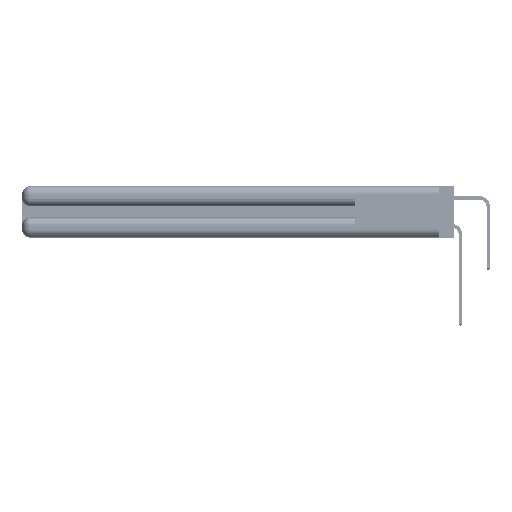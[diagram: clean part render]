
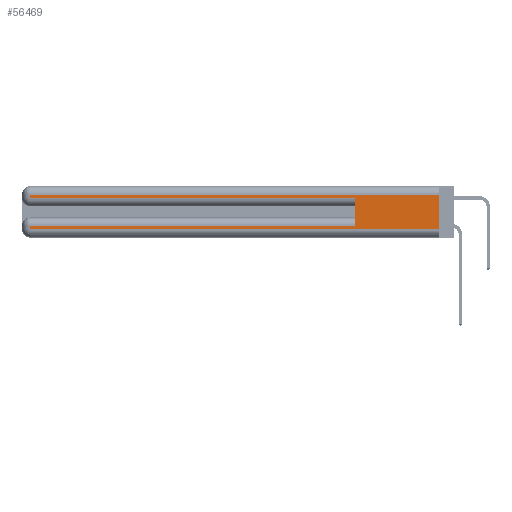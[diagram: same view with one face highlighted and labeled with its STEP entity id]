
A CAD part, left-side view. The second image highlights one B-rep face of the part: STEP entity #56469.
In plain terms, the highlighted planar face has unit normal (-1, 0, 0).
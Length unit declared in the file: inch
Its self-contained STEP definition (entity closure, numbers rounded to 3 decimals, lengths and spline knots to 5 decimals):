
#226 = VECTOR ( 'NONE', #22528, 39.37008 ) ;
#577 = CARTESIAN_POINT ( 'NONE',  ( 0., 0., 0.31 ) ) ;
#932 = CARTESIAN_POINT ( 'NONE',  ( 0., 0., 0.31 ) ) ;
#1440 = ORIENTED_EDGE ( 'NONE', *, *, #50047, .T. ) ;
#1702 = DIRECTION ( 'NONE',  ( 0., 0., -1. ) ) ;
#3631 = CARTESIAN_POINT ( 'NONE',  ( 0., 2.94, 0.37 ) ) ;
#4319 = DIRECTION ( 'NONE',  ( 0., -1., 0. ) ) ;
#5588 = ORIENTED_EDGE ( 'NONE', *, *, #55265, .F. ) ;
#5700 = DIRECTION ( 'NONE',  ( 0., 1., 0. ) ) ;
#7514 = CARTESIAN_POINT ( 'NONE',  ( 0., 0.6, 0.085 ) ) ;
#7896 = VERTEX_POINT ( 'NONE', #24627 ) ;
#8628 = DIRECTION ( 'NONE',  ( 0., 0., -1. ) ) ;
#9315 = CARTESIAN_POINT ( 'NONE',  ( 0., 2.94, 0.31 ) ) ;
#9508 = VERTEX_POINT ( 'NONE', #26844 ) ;
#10034 = EDGE_CURVE ( 'NONE', #7896, #24308, #26933, .T. ) ;
#10511 = LINE ( 'NONE', #32100, #226 ) ;
#11722 = CARTESIAN_POINT ( 'NONE',  ( 0., 0., 0.085 ) ) ;
#12884 = EDGE_CURVE ( 'NONE', #9508, #7896, #23349, .T. ) ;
#13428 = EDGE_LOOP ( 'NONE', ( #24247, #50853, #1440, #20833, #5588, #23877, #18763, #14285 ) ) ;
#14285 = ORIENTED_EDGE ( 'NONE', *, *, #10034, .T. ) ;
#14536 = FACE_OUTER_BOUND ( 'NONE', #13428, .T. ) ;
#16169 = VERTEX_POINT ( 'NONE', #32330 ) ;
#18763 = ORIENTED_EDGE ( 'NONE', *, *, #12884, .T. ) ;
#19368 = CARTESIAN_POINT ( 'NONE',  ( 0., 2.94, 0.37 ) ) ;
#20833 = ORIENTED_EDGE ( 'NONE', *, *, #41409, .T. ) ;
#21423 = VECTOR ( 'NONE', #4319, 39.37008 ) ;
#22528 = DIRECTION ( 'NONE',  ( 0., 0., 1. ) ) ;
#23249 = VECTOR ( 'NONE', #35732, 39.37008 ) ;
#23349 = LINE ( 'NONE', #3631, #53613 ) ;
#23877 = ORIENTED_EDGE ( 'NONE', *, *, #50041, .T. ) ;
#24247 = ORIENTED_EDGE ( 'NONE', *, *, #48035, .F. ) ;
#24308 = VERTEX_POINT ( 'NONE', #40683 ) ;
#24627 = CARTESIAN_POINT ( 'NONE',  ( 0., 2.94, 0.06 ) ) ;
#26844 = CARTESIAN_POINT ( 'NONE',  ( 0., 2.94, 0.085 ) ) ;
#26933 = LINE ( 'NONE', #43528, #21423 ) ;
#28744 = VERTEX_POINT ( 'NONE', #9315 ) ;
#29138 = DIRECTION ( 'NONE',  ( 0., 1., 0. ) ) ;
#29886 = VERTEX_POINT ( 'NONE', #39782 ) ;
#31624 = DIRECTION ( 'NONE',  ( 1., 0., 0. ) ) ;
#32100 = CARTESIAN_POINT ( 'NONE',  ( 0., 0.6, 0.145 ) ) ;
#32330 = CARTESIAN_POINT ( 'NONE',  ( 0., 0.6, 0.285 ) ) ;
#32557 = LINE ( 'NONE', #32590, #39495 ) ;
#32590 = CARTESIAN_POINT ( 'NONE',  ( 0., 0., 0.285 ) ) ;
#32706 = EDGE_CURVE ( 'NONE', #56368, #28744, #54175, .T. ) ;
#33718 = DIRECTION ( 'NONE',  ( 0., -1., 0. ) ) ;
#35732 = DIRECTION ( 'NONE',  ( 0., 0., -1. ) ) ;
#36448 = PLANE ( 'NONE',  #44457 ) ;
#37038 = LINE ( 'NONE', #53015, #23249 ) ;
#39495 = VECTOR ( 'NONE', #33718, 39.37008 ) ;
#39782 = CARTESIAN_POINT ( 'NONE',  ( 0., 2.94, 0.285 ) ) ;
#40683 = CARTESIAN_POINT ( 'NONE',  ( 0., 0., 0.06 ) ) ;
#41084 = CARTESIAN_POINT ( 'NONE',  ( 0., 0., 0.37 ) ) ;
#41409 = EDGE_CURVE ( 'NONE', #29886, #16169, #32557, .T. ) ;
#43075 = VECTOR ( 'NONE', #29138, 39.37008 ) ;
#43528 = CARTESIAN_POINT ( 'NONE',  ( 0., 0., 0.06 ) ) ;
#43911 = VECTOR ( 'NONE', #5700, 39.37008 ) ;
#44457 = AXIS2_PLACEMENT_3D ( 'NONE', #41084, #31624, #1702 ) ;
#46497 = LINE ( 'NONE', #19368, #50585 ) ;
#46653 = DIRECTION ( 'NONE',  ( 0., 0., -1. ) ) ;
#48035 = EDGE_CURVE ( 'NONE', #56368, #24308, #37038, .T. ) ;
#50041 = EDGE_CURVE ( 'NONE', #53754, #9508, #55382, .T. ) ;
#50047 = EDGE_CURVE ( 'NONE', #28744, #29886, #46497, .T. ) ;
#50585 = VECTOR ( 'NONE', #46653, 39.37008 ) ;
#50853 = ORIENTED_EDGE ( 'NONE', *, *, #32706, .T. ) ;
#53015 = CARTESIAN_POINT ( 'NONE',  ( 0., 0., 0.37 ) ) ;
#53613 = VECTOR ( 'NONE', #8628, 39.37008 ) ;
#53754 = VERTEX_POINT ( 'NONE', #7514 ) ;
#54175 = LINE ( 'NONE', #932, #43911 ) ;
#55265 = EDGE_CURVE ( 'NONE', #53754, #16169, #10511, .T. ) ;
#55382 = LINE ( 'NONE', #11722, #43075 ) ;
#56368 = VERTEX_POINT ( 'NONE', #577 ) ;
#56469 = ADVANCED_FACE ( 'NONE', ( #14536 ), #36448, .F. ) ;
